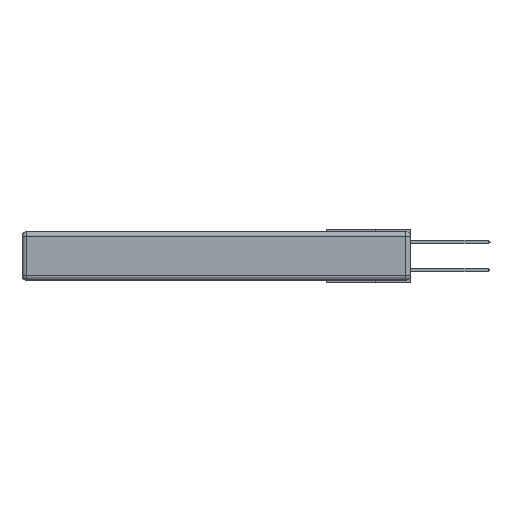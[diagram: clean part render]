
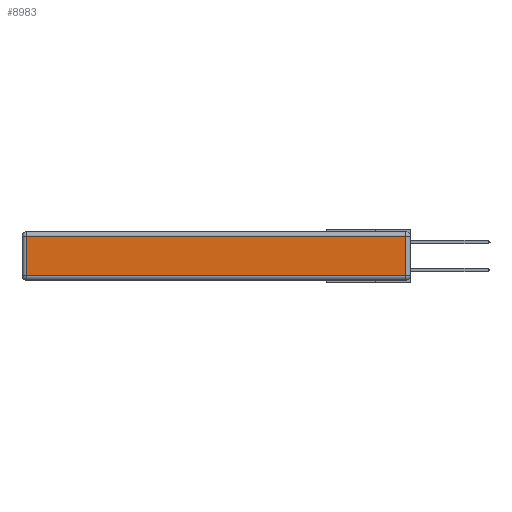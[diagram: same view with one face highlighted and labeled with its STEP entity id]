
A CAD part, left-side view. The second image highlights one B-rep face of the part: STEP entity #8983.
In plain terms, the highlighted planar face has unit normal (-1, 0, 0).
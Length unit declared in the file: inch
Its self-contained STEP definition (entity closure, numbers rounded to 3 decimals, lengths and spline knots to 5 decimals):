
#32 = CARTESIAN_POINT ( 'NONE',  ( 0., 2.72, -0.313 ) ) ;
#720 = ORIENTED_EDGE ( 'NONE', *, *, #10703, .T. ) ;
#884 = VERTEX_POINT ( 'NONE', #32 ) ;
#1332 = LINE ( 'NONE', #3434, #15614 ) ;
#2428 = LINE ( 'NONE', #10294, #9737 ) ;
#2709 = ORIENTED_EDGE ( 'NONE', *, *, #5490, .T. ) ;
#2732 = VECTOR ( 'NONE', #15230, 39.37008 ) ;
#3144 = CARTESIAN_POINT ( 'NONE',  ( 0., 0.03, -0.03 ) ) ;
#3434 = CARTESIAN_POINT ( 'NONE',  ( 0., 0.03, -0.343 ) ) ;
#4079 = DIRECTION ( 'NONE',  ( 0., 0., -1. ) ) ;
#4622 = EDGE_LOOP ( 'NONE', ( #2709, #8308, #14797, #720 ) ) ;
#5103 = EDGE_CURVE ( 'NONE', #9532, #9134, #10219, .T. ) ;
#5285 = CARTESIAN_POINT ( 'NONE',  ( 0., 0., -0.313 ) ) ;
#5320 = CARTESIAN_POINT ( 'NONE',  ( 0., 2.72, -0.03 ) ) ;
#5393 = VECTOR ( 'NONE', #8662, 39.37008 ) ;
#5490 = EDGE_CURVE ( 'NONE', #884, #8761, #7135, .T. ) ;
#7135 = LINE ( 'NONE', #5285, #2732 ) ;
#7508 = EDGE_CURVE ( 'NONE', #8761, #9532, #1332, .T. ) ;
#8308 = ORIENTED_EDGE ( 'NONE', *, *, #7508, .T. ) ;
#8662 = DIRECTION ( 'NONE',  ( 0., 1., 0. ) ) ;
#8761 = VERTEX_POINT ( 'NONE', #13409 ) ;
#8983 = ADVANCED_FACE ( 'NONE', ( #13449 ), #10929, .T. ) ;
#9134 = VERTEX_POINT ( 'NONE', #5320 ) ;
#9532 = VERTEX_POINT ( 'NONE', #3144 ) ;
#9737 = VECTOR ( 'NONE', #4079, 39.37008 ) ;
#10219 = LINE ( 'NONE', #14850, #5393 ) ;
#10294 = CARTESIAN_POINT ( 'NONE',  ( 0., 2.72, -0.343 ) ) ;
#10519 = AXIS2_PLACEMENT_3D ( 'NONE', #12402, #14941, #13759 ) ;
#10703 = EDGE_CURVE ( 'NONE', #9134, #884, #2428, .T. ) ;
#10929 = PLANE ( 'NONE',  #10519 ) ;
#12402 = CARTESIAN_POINT ( 'NONE',  ( 0., 0., -0.343 ) ) ;
#13257 = DIRECTION ( 'NONE',  ( 0., 0., 1. ) ) ;
#13409 = CARTESIAN_POINT ( 'NONE',  ( 0., 0.03, -0.313 ) ) ;
#13449 = FACE_OUTER_BOUND ( 'NONE', #4622, .T. ) ;
#13759 = DIRECTION ( 'NONE',  ( 0., 0., 1. ) ) ;
#14797 = ORIENTED_EDGE ( 'NONE', *, *, #5103, .T. ) ;
#14850 = CARTESIAN_POINT ( 'NONE',  ( 0., 2.75, -0.03 ) ) ;
#14941 = DIRECTION ( 'NONE',  ( -1., 0., 0. ) ) ;
#15230 = DIRECTION ( 'NONE',  ( 0., -1., 0. ) ) ;
#15614 = VECTOR ( 'NONE', #13257, 39.37008 ) ;
